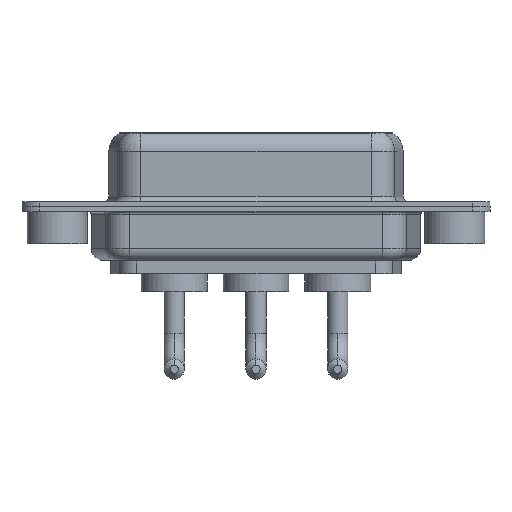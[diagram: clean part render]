
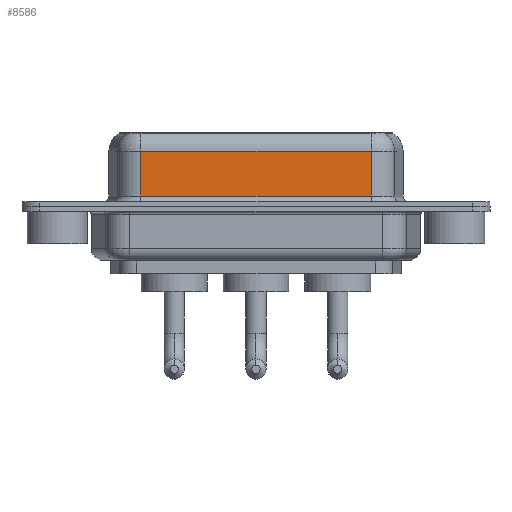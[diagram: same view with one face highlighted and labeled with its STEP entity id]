
A CAD part, front view. The second image highlights one B-rep face of the part: STEP entity #8586.
In plain terms, the highlighted planar face has unit normal (0, -1, 0).
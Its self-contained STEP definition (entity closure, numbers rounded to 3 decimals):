
#19 = VERTEX_POINT ( 'NONE', #4725 ) ;
#572 = DIRECTION ( 'NONE',  ( 0., 1., 0. ) ) ;
#847 = CARTESIAN_POINT ( 'NONE',  ( 26.287, -3.95, 4.65 ) ) ;
#863 = DIRECTION ( 'NONE',  ( 0., 0., -1. ) ) ;
#870 = ORIENTED_EDGE ( 'NONE', *, *, #3975, .T. ) ;
#1053 = LINE ( 'NONE', #6547, #4828 ) ;
#1208 = EDGE_CURVE ( 'NONE', #6171, #19, #7743, .T. ) ;
#1466 = CARTESIAN_POINT ( 'NONE',  ( 26.287, -3.95, 6.4 ) ) ;
#1799 = VECTOR ( 'NONE', #2853, 1000. ) ;
#1891 = ORIENTED_EDGE ( 'NONE', *, *, #6792, .T. ) ;
#1909 = ORIENTED_EDGE ( 'NONE', *, *, #1208, .T. ) ;
#2289 = DIRECTION ( 'NONE',  ( -1., 0., 0. ) ) ;
#2853 = DIRECTION ( 'NONE',  ( 0., 0., -1. ) ) ;
#2916 = LINE ( 'NONE', #8616, #1799 ) ;
#2957 = DIRECTION ( 'NONE',  ( 1., 0., 0. ) ) ;
#3025 = LINE ( 'NONE', #4136, #8794 ) ;
#3044 = CARTESIAN_POINT ( 'NONE',  ( 26.287, -3.95, 4.65 ) ) ;
#3512 = VERTEX_POINT ( 'NONE', #6461 ) ;
#3975 = EDGE_CURVE ( 'NONE', #19, #3512, #1053, .T. ) ;
#3978 = VECTOR ( 'NONE', #2289, 1000. ) ;
#4136 = CARTESIAN_POINT ( 'NONE',  ( 26.287, -3.95, 0.9 ) ) ;
#4680 = EDGE_LOOP ( 'NONE', ( #11247, #1909, #870, #1891 ) ) ;
#4725 = CARTESIAN_POINT ( 'NONE',  ( 7.013, -3.95, 4.65 ) ) ;
#4828 = VECTOR ( 'NONE', #863, 1000. ) ;
#5384 = DIRECTION ( 'NONE',  ( 0., 0., 1. ) ) ;
#6171 = VERTEX_POINT ( 'NONE', #847 ) ;
#6199 = EDGE_CURVE ( 'NONE', #6171, #8408, #2916, .T. ) ;
#6461 = CARTESIAN_POINT ( 'NONE',  ( 7.013, -3.95, 0.9 ) ) ;
#6547 = CARTESIAN_POINT ( 'NONE',  ( 7.013, -3.95, 6.4 ) ) ;
#6792 = EDGE_CURVE ( 'NONE', #3512, #8408, #3025, .T. ) ;
#7743 = LINE ( 'NONE', #3044, #3978 ) ;
#8161 = FACE_OUTER_BOUND ( 'NONE', #4680, .T. ) ;
#8295 = PLANE ( 'NONE',  #10450 ) ;
#8408 = VERTEX_POINT ( 'NONE', #9442 ) ;
#8586 = ADVANCED_FACE ( 'NONE', ( #8161 ), #8295, .F. ) ;
#8616 = CARTESIAN_POINT ( 'NONE',  ( 26.287, -3.95, 6.4 ) ) ;
#8794 = VECTOR ( 'NONE', #2957, 1000. ) ;
#9442 = CARTESIAN_POINT ( 'NONE',  ( 26.287, -3.95, 0.9 ) ) ;
#10450 = AXIS2_PLACEMENT_3D ( 'NONE', #1466, #572, #5384 ) ;
#11247 = ORIENTED_EDGE ( 'NONE', *, *, #6199, .F. ) ;
